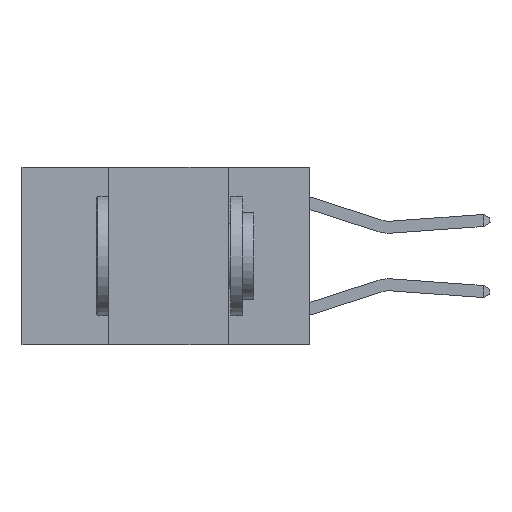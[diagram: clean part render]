
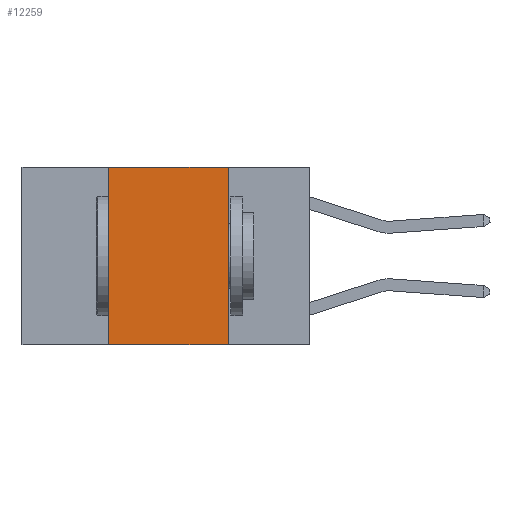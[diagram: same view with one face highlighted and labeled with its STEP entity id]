
A CAD part, left-side view. The second image highlights one B-rep face of the part: STEP entity #12259.
In plain terms, the highlighted planar face has unit normal (-1, 0, 0).
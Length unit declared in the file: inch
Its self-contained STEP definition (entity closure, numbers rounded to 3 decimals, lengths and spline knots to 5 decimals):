
#220 = ORIENTED_EDGE ( 'NONE', *, *, #5876, .F. ) ;
#295 = DIRECTION ( 'NONE',  ( 0., 0., -1. ) ) ;
#724 = VERTEX_POINT ( 'NONE', #9982 ) ;
#1318 = EDGE_CURVE ( 'NONE', #724, #9679, #4191, .T. ) ;
#1526 = VERTEX_POINT ( 'NONE', #1992 ) ;
#1992 = CARTESIAN_POINT ( 'NONE',  ( 0., 0.17, 0. ) ) ;
#2210 = DIRECTION ( 'NONE',  ( 0., -1., 0. ) ) ;
#3086 = DIRECTION ( 'NONE',  ( 0., 0., -1. ) ) ;
#3850 = VECTOR ( 'NONE', #12522, 39.37008 ) ;
#4191 = LINE ( 'NONE', #4762, #3850 ) ;
#4194 = CARTESIAN_POINT ( 'NONE',  ( 0., 0.17, 0. ) ) ;
#4762 = CARTESIAN_POINT ( 'NONE',  ( 0., 0.6, -0.37 ) ) ;
#5866 = ORIENTED_EDGE ( 'NONE', *, *, #12996, .F. ) ;
#5876 = EDGE_CURVE ( 'NONE', #9634, #1526, #8982, .T. ) ;
#5991 = VECTOR ( 'NONE', #2210, 39.37008 ) ;
#6222 = PLANE ( 'NONE',  #7228 ) ;
#6270 = DIRECTION ( 'NONE',  ( 0., 0., 1. ) ) ;
#7228 = AXIS2_PLACEMENT_3D ( 'NONE', #11733, #7352, #295 ) ;
#7352 = DIRECTION ( 'NONE',  ( 1., 0., 0. ) ) ;
#7390 = LINE ( 'NONE', #12932, #10390 ) ;
#7700 = CARTESIAN_POINT ( 'NONE',  ( 0., 0.17, -0.37 ) ) ;
#7767 = FACE_OUTER_BOUND ( 'NONE', #12292, .T. ) ;
#8982 = LINE ( 'NONE', #9014, #5991 ) ;
#9014 = CARTESIAN_POINT ( 'NONE',  ( 0., 0.6, 0. ) ) ;
#9538 = ORIENTED_EDGE ( 'NONE', *, *, #14453, .F. ) ;
#9634 = VERTEX_POINT ( 'NONE', #10989 ) ;
#9679 = VERTEX_POINT ( 'NONE', #7700 ) ;
#9982 = CARTESIAN_POINT ( 'NONE',  ( 0., 0.42, -0.37 ) ) ;
#10241 = LINE ( 'NONE', #4194, #12136 ) ;
#10390 = VECTOR ( 'NONE', #6270, 39.37008 ) ;
#10989 = CARTESIAN_POINT ( 'NONE',  ( 0., 0.42, 0. ) ) ;
#11733 = CARTESIAN_POINT ( 'NONE',  ( 0., 0.6, 0. ) ) ;
#12136 = VECTOR ( 'NONE', #3086, 39.37008 ) ;
#12259 = ADVANCED_FACE ( 'NONE', ( #7767 ), #6222, .F. ) ;
#12292 = EDGE_LOOP ( 'NONE', ( #5866, #220, #9538, #12479 ) ) ;
#12479 = ORIENTED_EDGE ( 'NONE', *, *, #1318, .T. ) ;
#12522 = DIRECTION ( 'NONE',  ( 0., -1., 0. ) ) ;
#12932 = CARTESIAN_POINT ( 'NONE',  ( 0., 0.42, 0. ) ) ;
#12996 = EDGE_CURVE ( 'NONE', #1526, #9679, #10241, .T. ) ;
#14453 = EDGE_CURVE ( 'NONE', #724, #9634, #7390, .T. ) ;
